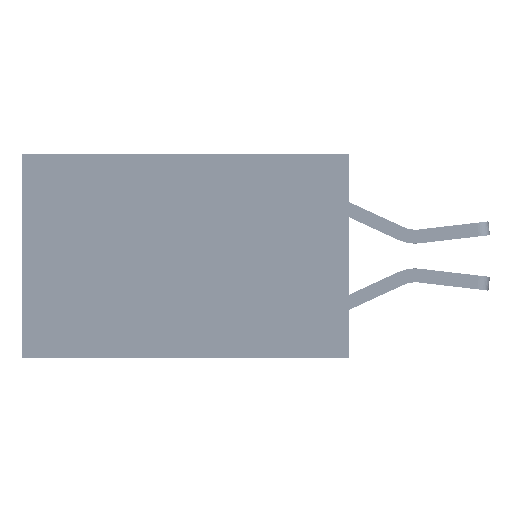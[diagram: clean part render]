
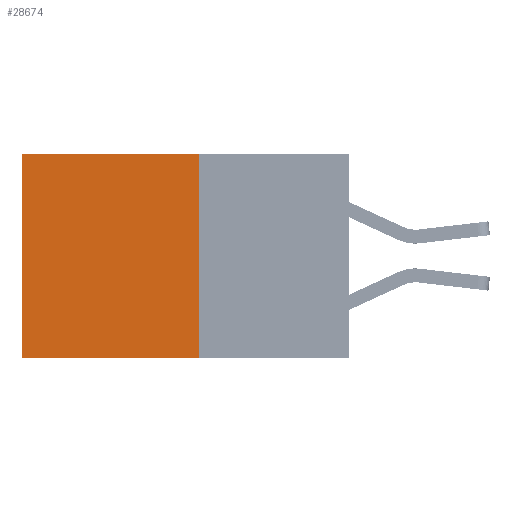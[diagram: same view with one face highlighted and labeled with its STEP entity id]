
A CAD part, left-side view. The second image highlights one B-rep face of the part: STEP entity #28674.
In plain terms, the highlighted planar face has unit normal (-1, 0, 0).
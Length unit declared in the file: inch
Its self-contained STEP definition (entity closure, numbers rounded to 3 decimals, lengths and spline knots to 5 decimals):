
#1601 = VERTEX_POINT ( 'NONE', #6746 ) ;
#1921 = EDGE_LOOP ( 'NONE', ( #25852, #2371, #9236, #28769 ) ) ;
#2113 = DIRECTION ( 'NONE',  ( 0., 1., 0. ) ) ;
#2371 = ORIENTED_EDGE ( 'NONE', *, *, #3452, .F. ) ;
#2406 = PLANE ( 'NONE',  #6165 ) ;
#2426 = LINE ( 'NONE', #22211, #22746 ) ;
#2638 = CARTESIAN_POINT ( 'NONE',  ( 0.277, 0.59, 0. ) ) ;
#3452 = EDGE_CURVE ( 'NONE', #30551, #33168, #2426, .T. ) ;
#6165 = AXIS2_PLACEMENT_3D ( 'NONE', #20936, #23563, #7786 ) ;
#6746 = CARTESIAN_POINT ( 'NONE',  ( 0.277, 0.27, 0. ) ) ;
#7068 = DIRECTION ( 'NONE',  ( 0., 0., -1. ) ) ;
#7786 = DIRECTION ( 'NONE',  ( 0., 0., -1. ) ) ;
#9236 = ORIENTED_EDGE ( 'NONE', *, *, #16871, .F. ) ;
#12395 = CARTESIAN_POINT ( 'NONE',  ( 0.277, 0.59, -0.37 ) ) ;
#13083 = VERTEX_POINT ( 'NONE', #2638 ) ;
#16871 = EDGE_CURVE ( 'NONE', #1601, #30551, #32357, .T. ) ;
#19142 = CARTESIAN_POINT ( 'NONE',  ( 0.277, 0.59, -0.37 ) ) ;
#19347 = FACE_OUTER_BOUND ( 'NONE', #1921, .T. ) ;
#19721 = CARTESIAN_POINT ( 'NONE',  ( 0.277, 0.27, -0.37 ) ) ;
#20936 = CARTESIAN_POINT ( 'NONE',  ( 0.277, 0.27, -0.37 ) ) ;
#21347 = DIRECTION ( 'NONE',  ( 0., 0., -1. ) ) ;
#21484 = DIRECTION ( 'NONE',  ( 0., 1., 0. ) ) ;
#22211 = CARTESIAN_POINT ( 'NONE',  ( 0.277, 0.27, -0.37 ) ) ;
#22746 = VECTOR ( 'NONE', #21484, 39.37008 ) ;
#23267 = CARTESIAN_POINT ( 'NONE',  ( 0.277, 0.27, 0. ) ) ;
#23563 = DIRECTION ( 'NONE',  ( 1., 0., 0. ) ) ;
#25852 = ORIENTED_EDGE ( 'NONE', *, *, #30090, .T. ) ;
#26531 = CARTESIAN_POINT ( 'NONE',  ( 0.277, 0.27, -0.37 ) ) ;
#26971 = LINE ( 'NONE', #23267, #32969 ) ;
#28128 = VECTOR ( 'NONE', #7068, 39.37008 ) ;
#28674 = ADVANCED_FACE ( 'NONE', ( #19347 ), #2406, .F. ) ;
#28769 = ORIENTED_EDGE ( 'NONE', *, *, #29950, .T. ) ;
#28919 = LINE ( 'NONE', #12395, #28128 ) ;
#29950 = EDGE_CURVE ( 'NONE', #1601, #13083, #26971, .T. ) ;
#30090 = EDGE_CURVE ( 'NONE', #13083, #33168, #28919, .T. ) ;
#30551 = VERTEX_POINT ( 'NONE', #19721 ) ;
#31552 = VECTOR ( 'NONE', #21347, 39.37008 ) ;
#32357 = LINE ( 'NONE', #26531, #31552 ) ;
#32969 = VECTOR ( 'NONE', #2113, 39.37008 ) ;
#33168 = VERTEX_POINT ( 'NONE', #19142 ) ;
